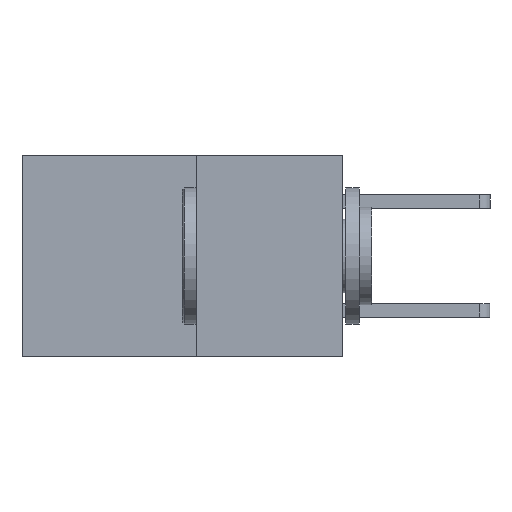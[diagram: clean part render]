
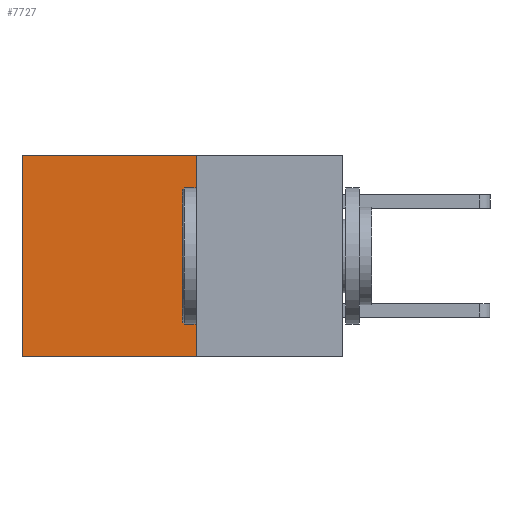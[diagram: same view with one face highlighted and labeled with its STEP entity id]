
A CAD part, left-side view. The second image highlights one B-rep face of the part: STEP entity #7727.
In plain terms, the highlighted planar face has unit normal (-1, 0, 0).
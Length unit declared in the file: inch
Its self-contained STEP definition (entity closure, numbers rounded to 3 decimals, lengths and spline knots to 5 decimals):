
#118 = VERTEX_POINT ( 'NONE', #7408 ) ;
#221 = VERTEX_POINT ( 'NONE', #7270 ) ;
#409 = VECTOR ( 'NONE', #6067, 39.37008 ) ;
#784 = CARTESIAN_POINT ( 'NONE',  ( 0.277, 0.27, -0.37 ) ) ;
#1130 = LINE ( 'NONE', #8059, #3972 ) ;
#1481 = DIRECTION ( 'NONE',  ( 1., 0., 0. ) ) ;
#2285 = LINE ( 'NONE', #2546, #7267 ) ;
#2341 = EDGE_CURVE ( 'NONE', #2670, #118, #1130, .T. ) ;
#2497 = LINE ( 'NONE', #6810, #409 ) ;
#2546 = CARTESIAN_POINT ( 'NONE',  ( 0.277, 0.27, -0.37 ) ) ;
#2670 = VERTEX_POINT ( 'NONE', #6053 ) ;
#2683 = DIRECTION ( 'NONE',  ( 0., 0., -1. ) ) ;
#2715 = LINE ( 'NONE', #6669, #7464 ) ;
#2825 = DIRECTION ( 'NONE',  ( 0., 1., 0. ) ) ;
#3684 = FACE_OUTER_BOUND ( 'NONE', #5349, .T. ) ;
#3701 = EDGE_CURVE ( 'NONE', #3935, #221, #2715, .T. ) ;
#3736 = EDGE_CURVE ( 'NONE', #3935, #2670, #2497, .T. ) ;
#3935 = VERTEX_POINT ( 'NONE', #4666 ) ;
#3972 = VECTOR ( 'NONE', #2683, 39.37008 ) ;
#4666 = CARTESIAN_POINT ( 'NONE',  ( 0.277, 0.27, 0. ) ) ;
#4686 = PLANE ( 'NONE',  #6391 ) ;
#4851 = EDGE_CURVE ( 'NONE', #221, #118, #2285, .T. ) ;
#4954 = ORIENTED_EDGE ( 'NONE', *, *, #2341, .T. ) ;
#5349 = EDGE_LOOP ( 'NONE', ( #4954, #6958, #6682, #6255 ) ) ;
#5945 = DIRECTION ( 'NONE',  ( 0., 0., -1. ) ) ;
#6053 = CARTESIAN_POINT ( 'NONE',  ( 0.277, 0.59, 0. ) ) ;
#6067 = DIRECTION ( 'NONE',  ( 0., 1., 0. ) ) ;
#6255 = ORIENTED_EDGE ( 'NONE', *, *, #3736, .T. ) ;
#6391 = AXIS2_PLACEMENT_3D ( 'NONE', #784, #1481, #5945 ) ;
#6669 = CARTESIAN_POINT ( 'NONE',  ( 0.277, 0.27, -0.37 ) ) ;
#6682 = ORIENTED_EDGE ( 'NONE', *, *, #3701, .F. ) ;
#6716 = DIRECTION ( 'NONE',  ( 0., 0., -1. ) ) ;
#6810 = CARTESIAN_POINT ( 'NONE',  ( 0.277, 0.27, 0. ) ) ;
#6958 = ORIENTED_EDGE ( 'NONE', *, *, #4851, .F. ) ;
#7267 = VECTOR ( 'NONE', #2825, 39.37008 ) ;
#7270 = CARTESIAN_POINT ( 'NONE',  ( 0.277, 0.27, -0.37 ) ) ;
#7408 = CARTESIAN_POINT ( 'NONE',  ( 0.277, 0.59, -0.37 ) ) ;
#7464 = VECTOR ( 'NONE', #6716, 39.37008 ) ;
#7727 = ADVANCED_FACE ( 'NONE', ( #3684 ), #4686, .F. ) ;
#8059 = CARTESIAN_POINT ( 'NONE',  ( 0.277, 0.59, -0.37 ) ) ;
